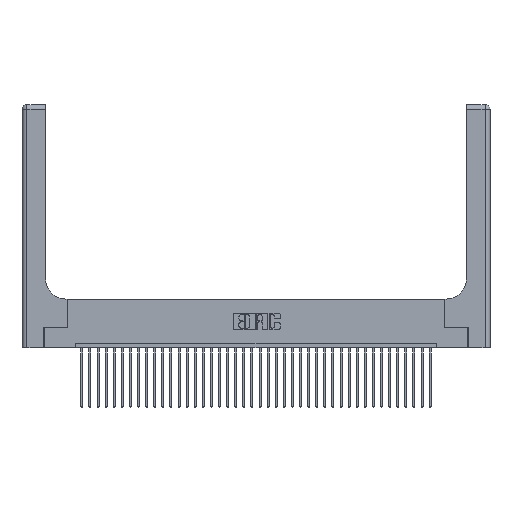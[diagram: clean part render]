
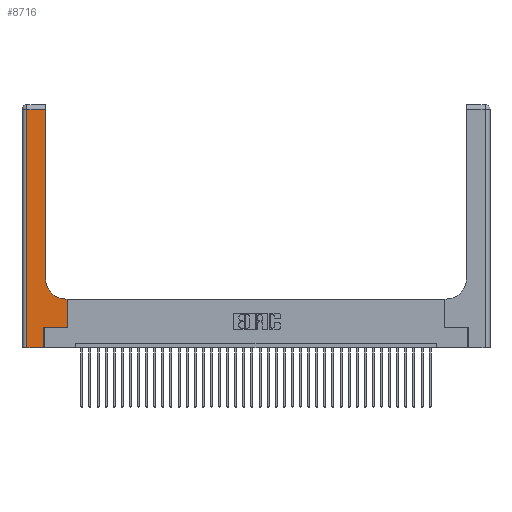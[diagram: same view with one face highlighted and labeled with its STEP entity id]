
A CAD part, top view. The second image highlights one B-rep face of the part: STEP entity #8716.
In plain terms, the highlighted planar face has unit normal (0, 0, 1).
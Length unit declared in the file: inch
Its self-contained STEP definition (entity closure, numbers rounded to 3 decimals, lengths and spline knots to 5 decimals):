
#459 = PLANE ( 'NONE',  #5631 ) ;
#2289 = VECTOR ( 'NONE', #18788, 39.37008 ) ;
#2311 = VERTEX_POINT ( 'NONE', #7051 ) ;
#3230 = DIRECTION ( 'NONE',  ( -1., 0., 0. ) ) ;
#3419 = VECTOR ( 'NONE', #36739, 39.37008 ) ;
#3579 = VERTEX_POINT ( 'NONE', #9974 ) ;
#3699 = DIRECTION ( 'NONE',  ( 0., -1., 0. ) ) ;
#4021 = ORIENTED_EDGE ( 'NONE', *, *, #37805, .T. ) ;
#4159 = ORIENTED_EDGE ( 'NONE', *, *, #36538, .T. ) ;
#5069 = VERTEX_POINT ( 'NONE', #11673 ) ;
#5246 = VERTEX_POINT ( 'NONE', #21260 ) ;
#5247 = VERTEX_POINT ( 'NONE', #30416 ) ;
#5379 = LINE ( 'NONE', #18328, #22429 ) ;
#5418 = CARTESIAN_POINT ( 'NONE',  ( 0.5585, 0.25, 0.37 ) ) ;
#5547 = CARTESIAN_POINT ( 'NONE',  ( 0.06, 0., 0.37 ) ) ;
#5631 = AXIS2_PLACEMENT_3D ( 'NONE', #12417, #32962, #18449 ) ;
#5652 = VECTOR ( 'NONE', #15217, 39.37008 ) ;
#5850 = EDGE_CURVE ( 'NONE', #2311, #3579, #18874, .T. ) ;
#7051 = CARTESIAN_POINT ( 'NONE',  ( 0.2915, 2.94, 0.37 ) ) ;
#7503 = EDGE_CURVE ( 'NONE', #5247, #5246, #20970, .T. ) ;
#7906 = AXIS2_PLACEMENT_3D ( 'NONE', #10436, #22861, #8103 ) ;
#8103 = DIRECTION ( 'NONE',  ( 1., 0., 0. ) ) ;
#8487 = EDGE_CURVE ( 'NONE', #5246, #17045, #34261, .T. ) ;
#8716 = ADVANCED_FACE ( 'NONE', ( #24594 ), #459, .F. ) ;
#9325 = CARTESIAN_POINT ( 'NONE',  ( 0.269, 0.25, 0.37 ) ) ;
#9974 = CARTESIAN_POINT ( 'NONE',  ( 0.06, 2.94, 0.37 ) ) ;
#10398 = EDGE_LOOP ( 'NONE', ( #4021, #23141, #34220, #15359, #26099, #4159, #17785, #30486, #19183 ) ) ;
#10436 = CARTESIAN_POINT ( 'NONE',  ( 0.5415, 0.85, 0.37 ) ) ;
#10735 = VERTEX_POINT ( 'NONE', #5547 ) ;
#10899 = CARTESIAN_POINT ( 'NONE',  ( 0.2915, 0.85, 0.37 ) ) ;
#11673 = CARTESIAN_POINT ( 'NONE',  ( 0.269, 0.25, 0.37 ) ) ;
#12211 = EDGE_CURVE ( 'NONE', #10735, #27105, #25700, .T. ) ;
#12323 = CARTESIAN_POINT ( 'NONE',  ( 0.269, 0., 0.37 ) ) ;
#12417 = CARTESIAN_POINT ( 'NONE',  ( 0., 3., 0.37 ) ) ;
#13379 = VECTOR ( 'NONE', #18480, 39.37008 ) ;
#13496 = LINE ( 'NONE', #9325, #5652 ) ;
#13691 = EDGE_CURVE ( 'NONE', #3579, #10735, #5379, .T. ) ;
#14696 = CARTESIAN_POINT ( 'NONE',  ( 0.5585, 0.25, 0.37 ) ) ;
#14900 = CARTESIAN_POINT ( 'NONE',  ( 0.2915, 0.6, 0.37 ) ) ;
#15054 = EDGE_CURVE ( 'NONE', #27105, #5069, #30579, .T. ) ;
#15217 = DIRECTION ( 'NONE',  ( 1., 0., 0. ) ) ;
#15359 = ORIENTED_EDGE ( 'NONE', *, *, #12211, .T. ) ;
#15798 = CARTESIAN_POINT ( 'NONE',  ( 0.2915, 3., 0.37 ) ) ;
#15943 = CARTESIAN_POINT ( 'NONE',  ( 0.269, 0., 0.37 ) ) ;
#16118 = VECTOR ( 'NONE', #32917, 39.37008 ) ;
#17045 = VERTEX_POINT ( 'NONE', #10899 ) ;
#17785 = ORIENTED_EDGE ( 'NONE', *, *, #21297, .T. ) ;
#18328 = CARTESIAN_POINT ( 'NONE',  ( 0.06, 3., 0.37 ) ) ;
#18449 = DIRECTION ( 'NONE',  ( -1., 0., 0. ) ) ;
#18480 = DIRECTION ( 'NONE',  ( 0., 1., 0. ) ) ;
#18788 = DIRECTION ( 'NONE',  ( 1., 0., 0. ) ) ;
#18874 = LINE ( 'NONE', #35614, #16118 ) ;
#19183 = ORIENTED_EDGE ( 'NONE', *, *, #8487, .T. ) ;
#20501 = VECTOR ( 'NONE', #31925, 39.37008 ) ;
#20970 = LINE ( 'NONE', #14900, #25622 ) ;
#21260 = CARTESIAN_POINT ( 'NONE',  ( 0.5415, 0.6, 0.37 ) ) ;
#21297 = EDGE_CURVE ( 'NONE', #31203, #5247, #29268, .T. ) ;
#22429 = VECTOR ( 'NONE', #3699, 39.37008 ) ;
#22861 = DIRECTION ( 'NONE',  ( 0., 0., -1. ) ) ;
#23141 = ORIENTED_EDGE ( 'NONE', *, *, #5850, .T. ) ;
#24594 = FACE_OUTER_BOUND ( 'NONE', #10398, .T. ) ;
#24694 = CARTESIAN_POINT ( 'NONE',  ( 0., 0., 0.37 ) ) ;
#25622 = VECTOR ( 'NONE', #3230, 39.37008 ) ;
#25700 = LINE ( 'NONE', #24694, #2289 ) ;
#26099 = ORIENTED_EDGE ( 'NONE', *, *, #15054, .T. ) ;
#27105 = VERTEX_POINT ( 'NONE', #15943 ) ;
#29268 = LINE ( 'NONE', #14696, #20501 ) ;
#30416 = CARTESIAN_POINT ( 'NONE',  ( 0.5585, 0.6, 0.37 ) ) ;
#30486 = ORIENTED_EDGE ( 'NONE', *, *, #7503, .T. ) ;
#30579 = LINE ( 'NONE', #12323, #3419 ) ;
#31203 = VERTEX_POINT ( 'NONE', #5418 ) ;
#31925 = DIRECTION ( 'NONE',  ( 0., 1., 0. ) ) ;
#32177 = LINE ( 'NONE', #15798, #13379 ) ;
#32917 = DIRECTION ( 'NONE',  ( -1., 0., 0. ) ) ;
#32962 = DIRECTION ( 'NONE',  ( 0., 0., -1. ) ) ;
#34220 = ORIENTED_EDGE ( 'NONE', *, *, #13691, .T. ) ;
#34261 = CIRCLE ( 'NONE', #7906, 0.25 ) ;
#35614 = CARTESIAN_POINT ( 'NONE',  ( 0., 2.94, 0.37 ) ) ;
#36538 = EDGE_CURVE ( 'NONE', #5069, #31203, #13496, .T. ) ;
#36739 = DIRECTION ( 'NONE',  ( 0., 1., 0. ) ) ;
#37805 = EDGE_CURVE ( 'NONE', #17045, #2311, #32177, .T. ) ;
